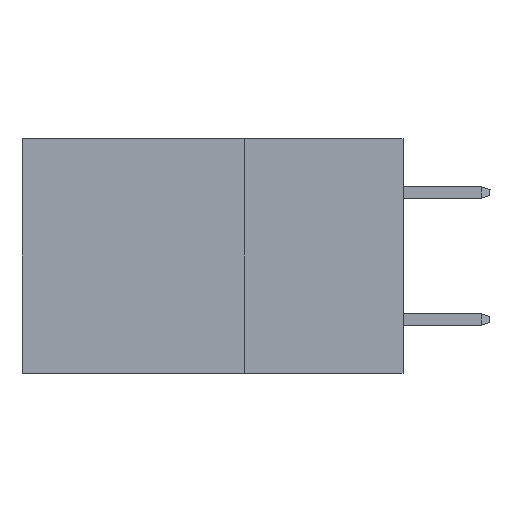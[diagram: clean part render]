
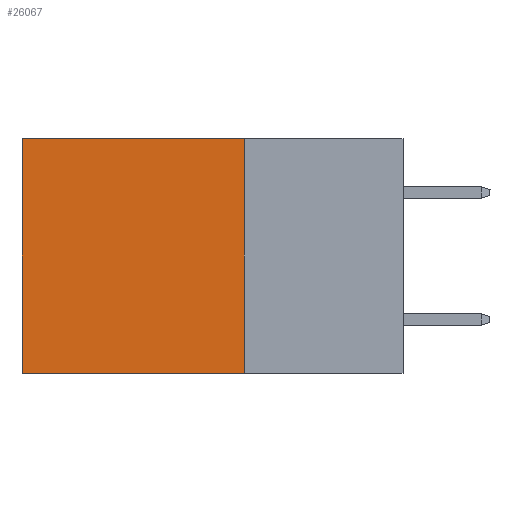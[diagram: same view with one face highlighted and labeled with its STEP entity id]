
A CAD part, left-side view. The second image highlights one B-rep face of the part: STEP entity #26067.
In plain terms, the highlighted planar face has unit normal (-1, 0, 0).
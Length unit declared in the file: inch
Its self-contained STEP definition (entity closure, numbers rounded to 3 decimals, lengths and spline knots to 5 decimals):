
#44 = DIRECTION ( 'NONE',  ( 0., 0., -1. ) ) ;
#3033 = EDGE_CURVE ( 'NONE', #20299, #24681, #4101, .T. ) ;
#3643 = DIRECTION ( 'NONE',  ( 0., 1., 0. ) ) ;
#3899 = FACE_OUTER_BOUND ( 'NONE', #13368, .T. ) ;
#3949 = CARTESIAN_POINT ( 'NONE',  ( 0.2875, 0.6, -0.37 ) ) ;
#4094 = DIRECTION ( 'NONE',  ( 1., 0., 0. ) ) ;
#4101 = LINE ( 'NONE', #22091, #24942 ) ;
#4279 = VERTEX_POINT ( 'NONE', #28221 ) ;
#9670 = VECTOR ( 'NONE', #3643, 39.37008 ) ;
#11653 = EDGE_CURVE ( 'NONE', #18398, #24681, #21291, .T. ) ;
#13368 = EDGE_LOOP ( 'NONE', ( #18385, #26270, #27965, #36765 ) ) ;
#13448 = DIRECTION ( 'NONE',  ( 0., 1., 0. ) ) ;
#15646 = LINE ( 'NONE', #28300, #9670 ) ;
#16598 = VECTOR ( 'NONE', #13448, 39.37008 ) ;
#18385 = ORIENTED_EDGE ( 'NONE', *, *, #3033, .T. ) ;
#18398 = VERTEX_POINT ( 'NONE', #37678 ) ;
#18932 = EDGE_CURVE ( 'NONE', #4279, #20299, #15646, .T. ) ;
#19853 = PLANE ( 'NONE',  #30488 ) ;
#20000 = CARTESIAN_POINT ( 'NONE',  ( 0.2875, 0.6, 0. ) ) ;
#20299 = VERTEX_POINT ( 'NONE', #20000 ) ;
#21291 = LINE ( 'NONE', #30570, #16598 ) ;
#22091 = CARTESIAN_POINT ( 'NONE',  ( 0.2875, 0.6, 0. ) ) ;
#22889 = DIRECTION ( 'NONE',  ( 0., 0., -1. ) ) ;
#24681 = VERTEX_POINT ( 'NONE', #3949 ) ;
#24942 = VECTOR ( 'NONE', #28176, 39.37008 ) ;
#26067 = ADVANCED_FACE ( 'NONE', ( #3899 ), #19853, .F. ) ;
#26270 = ORIENTED_EDGE ( 'NONE', *, *, #11653, .F. ) ;
#27525 = VECTOR ( 'NONE', #44, 39.37008 ) ;
#27965 = ORIENTED_EDGE ( 'NONE', *, *, #38985, .F. ) ;
#28105 = LINE ( 'NONE', #34082, #27525 ) ;
#28176 = DIRECTION ( 'NONE',  ( 0., 0., -1. ) ) ;
#28221 = CARTESIAN_POINT ( 'NONE',  ( 0.2875, 0.25, 0. ) ) ;
#28300 = CARTESIAN_POINT ( 'NONE',  ( 0.2875, 0.25, 0. ) ) ;
#30488 = AXIS2_PLACEMENT_3D ( 'NONE', #38298, #4094, #22889 ) ;
#30570 = CARTESIAN_POINT ( 'NONE',  ( 0.2875, 0.25, -0.37 ) ) ;
#34082 = CARTESIAN_POINT ( 'NONE',  ( 0.2875, 0.25, 0. ) ) ;
#36765 = ORIENTED_EDGE ( 'NONE', *, *, #18932, .T. ) ;
#37678 = CARTESIAN_POINT ( 'NONE',  ( 0.2875, 0.25, -0.37 ) ) ;
#38298 = CARTESIAN_POINT ( 'NONE',  ( 0.2875, 0.25, 0. ) ) ;
#38985 = EDGE_CURVE ( 'NONE', #4279, #18398, #28105, .T. ) ;
